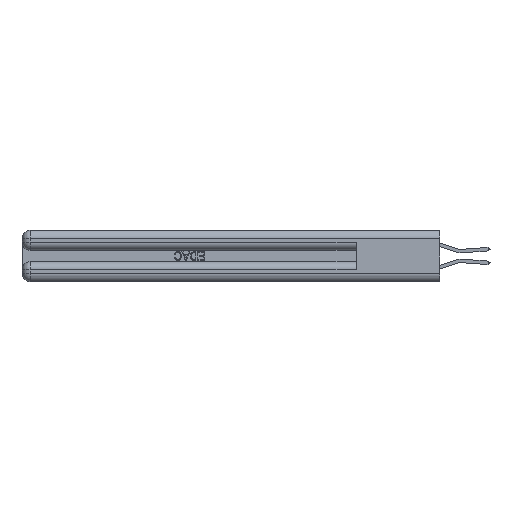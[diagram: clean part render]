
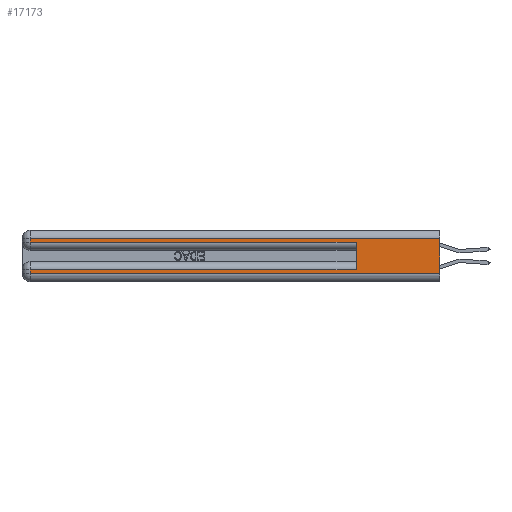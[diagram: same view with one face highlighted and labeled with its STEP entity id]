
A CAD part, left-side view. The second image highlights one B-rep face of the part: STEP entity #17173.
In plain terms, the highlighted planar face has unit normal (-1, 0, 0).
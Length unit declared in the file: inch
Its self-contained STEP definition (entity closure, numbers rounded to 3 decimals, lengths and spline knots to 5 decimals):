
#147 = EDGE_CURVE ( 'NONE', #10108, #30025, #17361, .T. ) ;
#195 = VECTOR ( 'NONE', #24666, 39.37008 ) ;
#1062 = LINE ( 'NONE', #10597, #16973 ) ;
#3612 = LINE ( 'NONE', #9757, #24450 ) ;
#4559 = ORIENTED_EDGE ( 'NONE', *, *, #30283, .T. ) ;
#4740 = LINE ( 'NONE', #43217, #40972 ) ;
#4744 = VERTEX_POINT ( 'NONE', #20915 ) ;
#5421 = CARTESIAN_POINT ( 'NONE',  ( 0., 0., 0.06 ) ) ;
#5993 = VERTEX_POINT ( 'NONE', #26690 ) ;
#6630 = EDGE_CURVE ( 'NONE', #38001, #19115, #3612, .T. ) ;
#7180 = ORIENTED_EDGE ( 'NONE', *, *, #38790, .F. ) ;
#7435 = CARTESIAN_POINT ( 'NONE',  ( 0., 0.6, 0.285 ) ) ;
#8266 = DIRECTION ( 'NONE',  ( 0., 0., 1. ) ) ;
#9519 = LINE ( 'NONE', #5421, #195 ) ;
#9757 = CARTESIAN_POINT ( 'NONE',  ( 0., 0., 0.31 ) ) ;
#10108 = VERTEX_POINT ( 'NONE', #39598 ) ;
#10597 = CARTESIAN_POINT ( 'NONE',  ( 0., 2.94, 0.37 ) ) ;
#11556 = ORIENTED_EDGE ( 'NONE', *, *, #22794, .T. ) ;
#11597 = ORIENTED_EDGE ( 'NONE', *, *, #25142, .T. ) ;
#12883 = ORIENTED_EDGE ( 'NONE', *, *, #38113, .F. ) ;
#12998 = ORIENTED_EDGE ( 'NONE', *, *, #147, .T. ) ;
#13167 = EDGE_LOOP ( 'NONE', ( #12883, #21913, #11597, #4559, #7180, #12998, #29474, #11556 ) ) ;
#13703 = DIRECTION ( 'NONE',  ( 0., 0., -1. ) ) ;
#14787 = DIRECTION ( 'NONE',  ( 0., 1., 0. ) ) ;
#15835 = VERTEX_POINT ( 'NONE', #7435 ) ;
#16954 = VERTEX_POINT ( 'NONE', #38450 ) ;
#16973 = VECTOR ( 'NONE', #43534, 39.37008 ) ;
#17036 = DIRECTION ( 'NONE',  ( 0., 0., -1. ) ) ;
#17173 = ADVANCED_FACE ( 'NONE', ( #18761 ), #24559, .F. ) ;
#17361 = LINE ( 'NONE', #28413, #35933 ) ;
#17935 = DIRECTION ( 'NONE',  ( 0., 1., 0. ) ) ;
#18685 = LINE ( 'NONE', #38315, #19219 ) ;
#18761 = FACE_OUTER_BOUND ( 'NONE', #13167, .T. ) ;
#19115 = VERTEX_POINT ( 'NONE', #35677 ) ;
#19219 = VECTOR ( 'NONE', #17036, 39.37008 ) ;
#19303 = EDGE_CURVE ( 'NONE', #30025, #16954, #1062, .T. ) ;
#19902 = LINE ( 'NONE', #28705, #30299 ) ;
#20915 = CARTESIAN_POINT ( 'NONE',  ( 0., 0., 0.06 ) ) ;
#21244 = CARTESIAN_POINT ( 'NONE',  ( 0., 0., 0.31 ) ) ;
#21913 = ORIENTED_EDGE ( 'NONE', *, *, #6630, .T. ) ;
#22613 = LINE ( 'NONE', #29746, #28602 ) ;
#22794 = EDGE_CURVE ( 'NONE', #16954, #4744, #9519, .T. ) ;
#24450 = VECTOR ( 'NONE', #17935, 39.37008 ) ;
#24559 = PLANE ( 'NONE',  #36502 ) ;
#24666 = DIRECTION ( 'NONE',  ( 0., -1., 0. ) ) ;
#25142 = EDGE_CURVE ( 'NONE', #19115, #5993, #18685, .T. ) ;
#26690 = CARTESIAN_POINT ( 'NONE',  ( 0., 2.94, 0.285 ) ) ;
#27711 = CARTESIAN_POINT ( 'NONE',  ( 0., 2.94, 0.085 ) ) ;
#27928 = DIRECTION ( 'NONE',  ( 1., 0., 0. ) ) ;
#28413 = CARTESIAN_POINT ( 'NONE',  ( 0., 0., 0.085 ) ) ;
#28602 = VECTOR ( 'NONE', #8266, 39.37008 ) ;
#28705 = CARTESIAN_POINT ( 'NONE',  ( 0., 0., 0.37 ) ) ;
#29474 = ORIENTED_EDGE ( 'NONE', *, *, #19303, .T. ) ;
#29746 = CARTESIAN_POINT ( 'NONE',  ( 0., 0.6, 0.145 ) ) ;
#30025 = VERTEX_POINT ( 'NONE', #27711 ) ;
#30283 = EDGE_CURVE ( 'NONE', #5993, #15835, #4740, .T. ) ;
#30299 = VECTOR ( 'NONE', #31644, 39.37008 ) ;
#31169 = CARTESIAN_POINT ( 'NONE',  ( 0., 0., 0.37 ) ) ;
#31644 = DIRECTION ( 'NONE',  ( 0., 0., -1. ) ) ;
#35677 = CARTESIAN_POINT ( 'NONE',  ( 0., 2.94, 0.31 ) ) ;
#35933 = VECTOR ( 'NONE', #14787, 39.37008 ) ;
#36502 = AXIS2_PLACEMENT_3D ( 'NONE', #31169, #27928, #13703 ) ;
#38001 = VERTEX_POINT ( 'NONE', #21244 ) ;
#38113 = EDGE_CURVE ( 'NONE', #38001, #4744, #19902, .T. ) ;
#38315 = CARTESIAN_POINT ( 'NONE',  ( 0., 2.94, 0.37 ) ) ;
#38450 = CARTESIAN_POINT ( 'NONE',  ( 0., 2.94, 0.06 ) ) ;
#38790 = EDGE_CURVE ( 'NONE', #10108, #15835, #22613, .T. ) ;
#39598 = CARTESIAN_POINT ( 'NONE',  ( 0., 0.6, 0.085 ) ) ;
#40972 = VECTOR ( 'NONE', #43053, 39.37008 ) ;
#43053 = DIRECTION ( 'NONE',  ( 0., -1., 0. ) ) ;
#43217 = CARTESIAN_POINT ( 'NONE',  ( 0., 0., 0.285 ) ) ;
#43534 = DIRECTION ( 'NONE',  ( 0., 0., -1. ) ) ;
